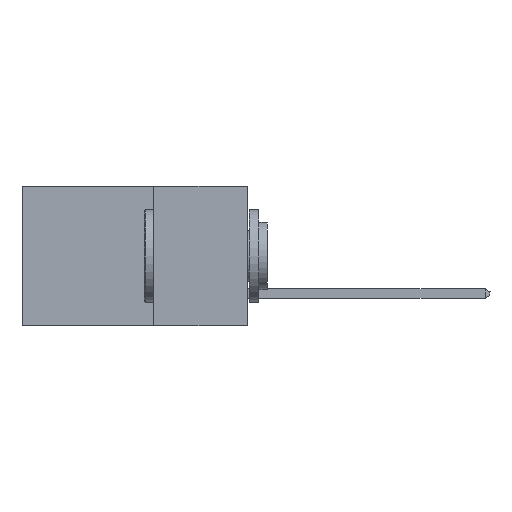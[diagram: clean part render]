
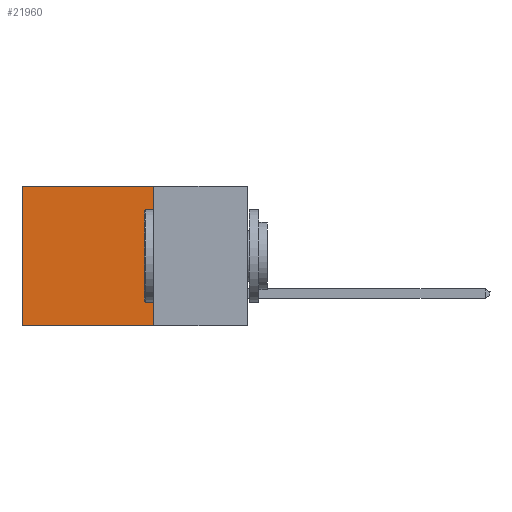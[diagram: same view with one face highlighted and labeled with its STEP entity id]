
A CAD part, left-side view. The second image highlights one B-rep face of the part: STEP entity #21960.
In plain terms, the highlighted planar face has unit normal (-1, 0, 0).
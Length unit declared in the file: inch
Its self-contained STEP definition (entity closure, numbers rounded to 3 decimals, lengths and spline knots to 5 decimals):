
#849 = ORIENTED_EDGE ( 'NONE', *, *, #25443, .F. ) ;
#952 = DIRECTION ( 'NONE',  ( 0., 0., -1. ) ) ;
#1290 = EDGE_LOOP ( 'NONE', ( #20190, #3874, #849, #23053 ) ) ;
#2005 = VECTOR ( 'NONE', #12516, 39.37008 ) ;
#3118 = CARTESIAN_POINT ( 'NONE',  ( 0.2615, 0.6, -0.37 ) ) ;
#3874 = ORIENTED_EDGE ( 'NONE', *, *, #8997, .F. ) ;
#5389 = DIRECTION ( 'NONE',  ( 0., 0., -1. ) ) ;
#5528 = CARTESIAN_POINT ( 'NONE',  ( 0.2615, 0.6, 0. ) ) ;
#6245 = VECTOR ( 'NONE', #5389, 39.37008 ) ;
#6693 = CARTESIAN_POINT ( 'NONE',  ( 0.2615, 0.25, 0. ) ) ;
#8430 = LINE ( 'NONE', #16392, #14112 ) ;
#8997 = EDGE_CURVE ( 'NONE', #21789, #25657, #16556, .T. ) ;
#9239 = PLANE ( 'NONE',  #22749 ) ;
#9319 = CARTESIAN_POINT ( 'NONE',  ( 0.2615, 0.6, -0.37 ) ) ;
#11448 = EDGE_CURVE ( 'NONE', #12737, #25657, #13750, .T. ) ;
#11520 = CARTESIAN_POINT ( 'NONE',  ( 0.2615, 0.25, 0. ) ) ;
#12516 = DIRECTION ( 'NONE',  ( 0., 1., 0. ) ) ;
#12737 = VERTEX_POINT ( 'NONE', #5528 ) ;
#13750 = LINE ( 'NONE', #9319, #6245 ) ;
#14079 = CARTESIAN_POINT ( 'NONE',  ( 0.2615, 0.25, -0.37 ) ) ;
#14112 = VECTOR ( 'NONE', #24643, 39.37008 ) ;
#16392 = CARTESIAN_POINT ( 'NONE',  ( 0.2615, 0.25, -0.37 ) ) ;
#16424 = CARTESIAN_POINT ( 'NONE',  ( 0.2615, 0.25, -0.37 ) ) ;
#16556 = LINE ( 'NONE', #16424, #2005 ) ;
#18905 = FACE_OUTER_BOUND ( 'NONE', #1290, .T. ) ;
#19492 = DIRECTION ( 'NONE',  ( 0., 1., 0. ) ) ;
#20190 = ORIENTED_EDGE ( 'NONE', *, *, #11448, .T. ) ;
#20941 = EDGE_CURVE ( 'NONE', #21454, #12737, #21463, .T. ) ;
#21454 = VERTEX_POINT ( 'NONE', #6693 ) ;
#21463 = LINE ( 'NONE', #11520, #24392 ) ;
#21789 = VERTEX_POINT ( 'NONE', #14079 ) ;
#21960 = ADVANCED_FACE ( 'NONE', ( #18905 ), #9239, .F. ) ;
#22749 = AXIS2_PLACEMENT_3D ( 'NONE', #23093, #24665, #952 ) ;
#23053 = ORIENTED_EDGE ( 'NONE', *, *, #20941, .T. ) ;
#23093 = CARTESIAN_POINT ( 'NONE',  ( 0.2615, 0.25, -0.37 ) ) ;
#24392 = VECTOR ( 'NONE', #19492, 39.37008 ) ;
#24643 = DIRECTION ( 'NONE',  ( 0., 0., -1. ) ) ;
#24665 = DIRECTION ( 'NONE',  ( 1., 0., 0. ) ) ;
#25443 = EDGE_CURVE ( 'NONE', #21454, #21789, #8430, .T. ) ;
#25657 = VERTEX_POINT ( 'NONE', #3118 ) ;
